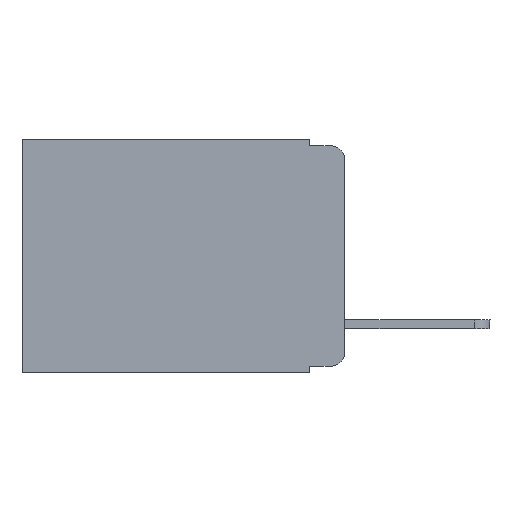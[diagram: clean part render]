
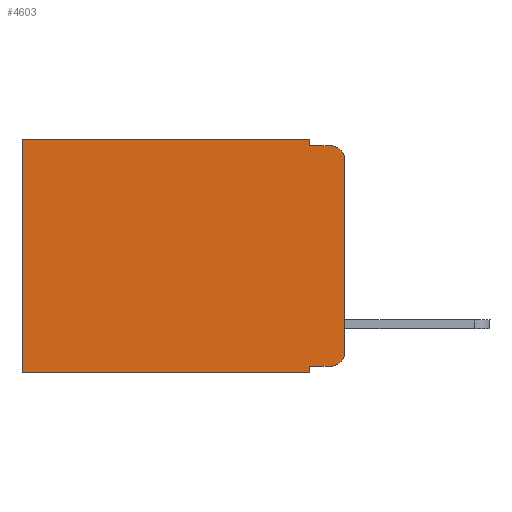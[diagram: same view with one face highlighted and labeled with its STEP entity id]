
A CAD part, left-side view. The second image highlights one B-rep face of the part: STEP entity #4603.
In plain terms, the highlighted planar face has unit normal (-1, 0, 0).
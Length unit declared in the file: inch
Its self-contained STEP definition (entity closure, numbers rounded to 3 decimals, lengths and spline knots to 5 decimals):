
#50 = LINE ( 'NONE', #6249, #1097 ) ;
#61 = EDGE_CURVE ( 'NONE', #4152, #8155, #5844, .T. ) ;
#160 = DIRECTION ( 'NONE',  ( 0., 0., -1. ) ) ;
#167 = EDGE_CURVE ( 'NONE', #4152, #7590, #3032, .T. ) ;
#202 = DIRECTION ( 'NONE',  ( 0., 1., 0. ) ) ;
#430 = ORIENTED_EDGE ( 'NONE', *, *, #602, .T. ) ;
#458 = VECTOR ( 'NONE', #8821, 39.37008 ) ;
#536 = CARTESIAN_POINT ( 'NONE',  ( 0.298, 0.051, -0.01 ) ) ;
#578 = EDGE_CURVE ( 'NONE', #8105, #9993, #4503, .T. ) ;
#602 = EDGE_CURVE ( 'NONE', #9920, #1728, #6619, .T. ) ;
#618 = DIRECTION ( 'NONE',  ( -1., 0., 0. ) ) ;
#621 = CARTESIAN_POINT ( 'NONE',  ( 0.298, 0.051, 0. ) ) ;
#675 = PLANE ( 'NONE',  #9949 ) ;
#821 = CARTESIAN_POINT ( 'NONE',  ( 0.298, 0., 0. ) ) ;
#1008 = DIRECTION ( 'NONE',  ( -1., 0., 0. ) ) ;
#1097 = VECTOR ( 'NONE', #4737, 39.37008 ) ;
#1143 = ORIENTED_EDGE ( 'NONE', *, *, #9088, .F. ) ;
#1430 = CARTESIAN_POINT ( 'NONE',  ( 0.298, 0.02, -0.333 ) ) ;
#1623 = LINE ( 'NONE', #4748, #8842 ) ;
#1722 = LINE ( 'NONE', #4078, #3408 ) ;
#1728 = VERTEX_POINT ( 'NONE', #6362 ) ;
#1767 = ORIENTED_EDGE ( 'NONE', *, *, #578, .F. ) ;
#1865 = CARTESIAN_POINT ( 'NONE',  ( 0.298, 0.051, -0.343 ) ) ;
#2156 = CARTESIAN_POINT ( 'NONE',  ( 0.298, 0.051, 0. ) ) ;
#2177 = DIRECTION ( 'NONE',  ( 0., 0., -1. ) ) ;
#2378 = VECTOR ( 'NONE', #6835, 39.37008 ) ;
#2890 = ORIENTED_EDGE ( 'NONE', *, *, #61, .T. ) ;
#2961 = FACE_OUTER_BOUND ( 'NONE', #6629, .T. ) ;
#3012 = DIRECTION ( 'NONE',  ( 1., 0., 0. ) ) ;
#3015 = EDGE_CURVE ( 'NONE', #7590, #8192, #1722, .T. ) ;
#3032 = LINE ( 'NONE', #2156, #9692 ) ;
#3374 = ORIENTED_EDGE ( 'NONE', *, *, #3015, .F. ) ;
#3408 = VECTOR ( 'NONE', #202, 39.37008 ) ;
#3597 = VECTOR ( 'NONE', #8415, 39.37008 ) ;
#3701 = DIRECTION ( 'NONE',  ( 0., 0., -1. ) ) ;
#3814 = ORIENTED_EDGE ( 'NONE', *, *, #9429, .F. ) ;
#3933 = EDGE_CURVE ( 'NONE', #9802, #8192, #9142, .T. ) ;
#4068 = EDGE_CURVE ( 'NONE', #8105, #9802, #1623, .T. ) ;
#4078 = CARTESIAN_POINT ( 'NONE',  ( 0.298, 0., -0.343 ) ) ;
#4152 = VERTEX_POINT ( 'NONE', #9026 ) ;
#4356 = CARTESIAN_POINT ( 'NONE',  ( 0.298, 0.051, -0.01 ) ) ;
#4420 = LINE ( 'NONE', #536, #3597 ) ;
#4433 = ORIENTED_EDGE ( 'NONE', *, *, #4942, .T. ) ;
#4503 = LINE ( 'NONE', #621, #2378 ) ;
#4603 = ADVANCED_FACE ( 'NONE', ( #2961 ), #675, .F. ) ;
#4737 = DIRECTION ( 'NONE',  ( 0., 0., -1. ) ) ;
#4746 = ORIENTED_EDGE ( 'NONE', *, *, #3933, .T. ) ;
#4748 = CARTESIAN_POINT ( 'NONE',  ( 0.298, 0., 0. ) ) ;
#4942 = EDGE_CURVE ( 'NONE', #8155, #7745, #7209, .T. ) ;
#4960 = VECTOR ( 'NONE', #2177, 39.37008 ) ;
#5113 = AXIS2_PLACEMENT_3D ( 'NONE', #6678, #618, #6021 ) ;
#5193 = CARTESIAN_POINT ( 'NONE',  ( 0.298, 0., -0.313 ) ) ;
#5418 = CARTESIAN_POINT ( 'NONE',  ( 0.298, 0.473, -0.343 ) ) ;
#5844 = LINE ( 'NONE', #8215, #458 ) ;
#6021 = DIRECTION ( 'NONE',  ( 0., 0., -1. ) ) ;
#6178 = DIRECTION ( 'NONE',  ( 0., 0., -1. ) ) ;
#6249 = CARTESIAN_POINT ( 'NONE',  ( 0.298, 0., 0. ) ) ;
#6362 = CARTESIAN_POINT ( 'NONE',  ( 0.298, 0.02, -0.01 ) ) ;
#6576 = CARTESIAN_POINT ( 'NONE',  ( 0.298, 0.473, 0. ) ) ;
#6619 = CIRCLE ( 'NONE', #8231, 0.02 ) ;
#6629 = EDGE_LOOP ( 'NONE', ( #1143, #430, #3814, #1767, #9658, #4746, #3374, #6889, #2890, #4433 ) ) ;
#6678 = CARTESIAN_POINT ( 'NONE',  ( 0.298, 0.02, -0.313 ) ) ;
#6835 = DIRECTION ( 'NONE',  ( 0., 0., -1. ) ) ;
#6889 = ORIENTED_EDGE ( 'NONE', *, *, #167, .F. ) ;
#7209 = CIRCLE ( 'NONE', #5113, 0.02 ) ;
#7481 = CARTESIAN_POINT ( 'NONE',  ( 0.298, 0., -0.03 ) ) ;
#7590 = VERTEX_POINT ( 'NONE', #1865 ) ;
#7745 = VERTEX_POINT ( 'NONE', #5193 ) ;
#7981 = CARTESIAN_POINT ( 'NONE',  ( 0.298, 0.02, -0.03 ) ) ;
#8105 = VERTEX_POINT ( 'NONE', #9957 ) ;
#8155 = VERTEX_POINT ( 'NONE', #1430 ) ;
#8192 = VERTEX_POINT ( 'NONE', #5418 ) ;
#8215 = CARTESIAN_POINT ( 'NONE',  ( 0.298, 0.051, -0.333 ) ) ;
#8231 = AXIS2_PLACEMENT_3D ( 'NONE', #7981, #1008, #160 ) ;
#8415 = DIRECTION ( 'NONE',  ( 0., -1., 0. ) ) ;
#8821 = DIRECTION ( 'NONE',  ( 0., -1., 0. ) ) ;
#8842 = VECTOR ( 'NONE', #9666, 39.37008 ) ;
#9026 = CARTESIAN_POINT ( 'NONE',  ( 0.298, 0.051, -0.333 ) ) ;
#9088 = EDGE_CURVE ( 'NONE', #9920, #7745, #50, .T. ) ;
#9142 = LINE ( 'NONE', #9293, #4960 ) ;
#9293 = CARTESIAN_POINT ( 'NONE',  ( 0.298, 0.473, 0. ) ) ;
#9429 = EDGE_CURVE ( 'NONE', #9993, #1728, #4420, .T. ) ;
#9658 = ORIENTED_EDGE ( 'NONE', *, *, #4068, .T. ) ;
#9666 = DIRECTION ( 'NONE',  ( 0., 1., 0. ) ) ;
#9692 = VECTOR ( 'NONE', #3701, 39.37008 ) ;
#9802 = VERTEX_POINT ( 'NONE', #6576 ) ;
#9920 = VERTEX_POINT ( 'NONE', #7481 ) ;
#9949 = AXIS2_PLACEMENT_3D ( 'NONE', #821, #3012, #6178 ) ;
#9957 = CARTESIAN_POINT ( 'NONE',  ( 0.298, 0.051, 0. ) ) ;
#9993 = VERTEX_POINT ( 'NONE', #4356 ) ;
